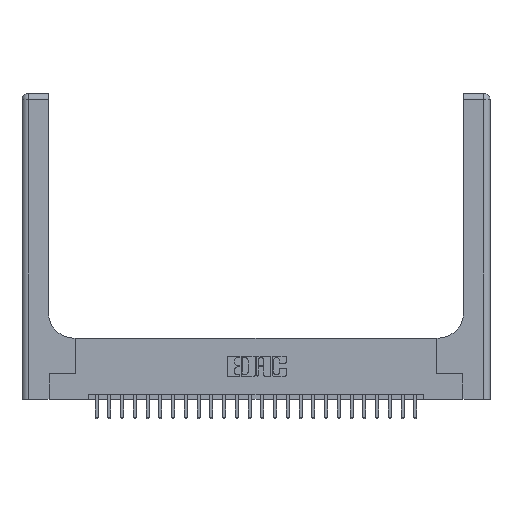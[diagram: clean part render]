
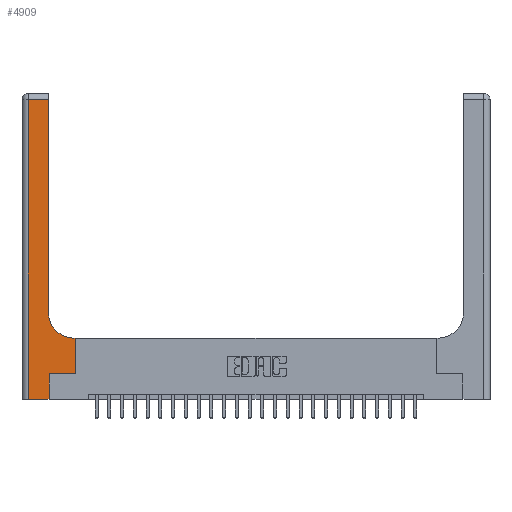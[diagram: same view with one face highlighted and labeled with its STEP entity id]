
A CAD part, top view. The second image highlights one B-rep face of the part: STEP entity #4909.
In plain terms, the highlighted planar face has unit normal (0, 0, 1).
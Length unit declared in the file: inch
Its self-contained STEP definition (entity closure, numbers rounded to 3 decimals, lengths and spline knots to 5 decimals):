
#277 = VERTEX_POINT ( 'NONE', #5348 ) ;
#520 = ORIENTED_EDGE ( 'NONE', *, *, #7861, .T. ) ;
#521 = EDGE_LOOP ( 'NONE', ( #4252, #520, #1349, #4184, #19137, #22256, #4974, #17528, #8665 ) ) ;
#565 = CIRCLE ( 'NONE', #12710, 0.25 ) ;
#1179 = EDGE_CURVE ( 'NONE', #9681, #13817, #15009, .T. ) ;
#1234 = LINE ( 'NONE', #13114, #2356 ) ;
#1349 = ORIENTED_EDGE ( 'NONE', *, *, #9516, .T. ) ;
#1449 = LINE ( 'NONE', #10674, #3967 ) ;
#2350 = EDGE_CURVE ( 'NONE', #13817, #20761, #4667, .T. ) ;
#2356 = VECTOR ( 'NONE', #8945, 39.37008 ) ;
#2433 = CARTESIAN_POINT ( 'NONE',  ( 0.265, 0., 0.37 ) ) ;
#2461 = CARTESIAN_POINT ( 'NONE',  ( 0.26, 2.94, 0.37 ) ) ;
#2468 = LINE ( 'NONE', #4597, #19761 ) ;
#2512 = EDGE_CURVE ( 'NONE', #20761, #14461, #565, .T. ) ;
#3032 = AXIS2_PLACEMENT_3D ( 'NONE', #6462, #14175, #21821 ) ;
#3412 = DIRECTION ( 'NONE',  ( 1., 0., 0. ) ) ;
#3967 = VECTOR ( 'NONE', #9165, 39.37008 ) ;
#4184 = ORIENTED_EDGE ( 'NONE', *, *, #15931, .T. ) ;
#4252 = ORIENTED_EDGE ( 'NONE', *, *, #15106, .T. ) ;
#4255 = VECTOR ( 'NONE', #4889, 39.37008 ) ;
#4597 = CARTESIAN_POINT ( 'NONE',  ( 0.06, 3., 0.37 ) ) ;
#4667 = LINE ( 'NONE', #8610, #19079 ) ;
#4889 = DIRECTION ( 'NONE',  ( 0., 1., 0. ) ) ;
#4909 = ADVANCED_FACE ( 'NONE', ( #14680 ), #23694, .F. ) ;
#4974 = ORIENTED_EDGE ( 'NONE', *, *, #1179, .T. ) ;
#5114 = CARTESIAN_POINT ( 'NONE',  ( 0.528, 0.25, 0.37 ) ) ;
#5348 = CARTESIAN_POINT ( 'NONE',  ( 0.06, 2.94, 0.37 ) ) ;
#5418 = CARTESIAN_POINT ( 'NONE',  ( 0.265, 0.25, 0.37 ) ) ;
#6462 = CARTESIAN_POINT ( 'NONE',  ( 0., 3., 0.37 ) ) ;
#6957 = DIRECTION ( 'NONE',  ( -1., 0., 0. ) ) ;
#7425 = DIRECTION ( 'NONE',  ( 0., 1., 0. ) ) ;
#7861 = EDGE_CURVE ( 'NONE', #8189, #277, #1234, .T. ) ;
#8189 = VERTEX_POINT ( 'NONE', #2461 ) ;
#8348 = VERTEX_POINT ( 'NONE', #12142 ) ;
#8610 = CARTESIAN_POINT ( 'NONE',  ( 0.26, 0.6, 0.37 ) ) ;
#8665 = ORIENTED_EDGE ( 'NONE', *, *, #2512, .T. ) ;
#8945 = DIRECTION ( 'NONE',  ( -1., 0., 0. ) ) ;
#9165 = DIRECTION ( 'NONE',  ( 1., 0., 0. ) ) ;
#9479 = DIRECTION ( 'NONE',  ( 0., 0., -1. ) ) ;
#9516 = EDGE_CURVE ( 'NONE', #277, #8348, #2468, .T. ) ;
#9681 = VERTEX_POINT ( 'NONE', #5114 ) ;
#10156 = LINE ( 'NONE', #15953, #14653 ) ;
#10674 = CARTESIAN_POINT ( 'NONE',  ( 0., 0., 0.37 ) ) ;
#10682 = CARTESIAN_POINT ( 'NONE',  ( 0.265, 0.25, 0.37 ) ) ;
#11364 = CARTESIAN_POINT ( 'NONE',  ( 0.51, 0.85, 0.37 ) ) ;
#12053 = DIRECTION ( 'NONE',  ( 0., 1., 0. ) ) ;
#12142 = CARTESIAN_POINT ( 'NONE',  ( 0.06, 0., 0.37 ) ) ;
#12207 = DIRECTION ( 'NONE',  ( 0., -1., 0. ) ) ;
#12710 = AXIS2_PLACEMENT_3D ( 'NONE', #11364, #9479, #3412 ) ;
#13114 = CARTESIAN_POINT ( 'NONE',  ( 0., 2.94, 0.37 ) ) ;
#13817 = VERTEX_POINT ( 'NONE', #21434 ) ;
#13982 = VECTOR ( 'NONE', #17362, 39.37008 ) ;
#14175 = DIRECTION ( 'NONE',  ( 0., 0., -1. ) ) ;
#14461 = VERTEX_POINT ( 'NONE', #16262 ) ;
#14653 = VECTOR ( 'NONE', #12053, 39.37008 ) ;
#14680 = FACE_OUTER_BOUND ( 'NONE', #521, .T. ) ;
#15009 = LINE ( 'NONE', #22634, #17061 ) ;
#15106 = EDGE_CURVE ( 'NONE', #14461, #8189, #10156, .T. ) ;
#15512 = CARTESIAN_POINT ( 'NONE',  ( 0.51, 0.6, 0.37 ) ) ;
#15931 = EDGE_CURVE ( 'NONE', #8348, #24026, #1449, .T. ) ;
#15953 = CARTESIAN_POINT ( 'NONE',  ( 0.26, 3., 0.37 ) ) ;
#16262 = CARTESIAN_POINT ( 'NONE',  ( 0.26, 0.85, 0.37 ) ) ;
#16788 = EDGE_CURVE ( 'NONE', #24026, #17146, #22136, .T. ) ;
#17061 = VECTOR ( 'NONE', #7425, 39.37008 ) ;
#17146 = VERTEX_POINT ( 'NONE', #10682 ) ;
#17362 = DIRECTION ( 'NONE',  ( 1., 0., 0. ) ) ;
#17528 = ORIENTED_EDGE ( 'NONE', *, *, #2350, .T. ) ;
#18492 = CARTESIAN_POINT ( 'NONE',  ( 0.265, 0., 0.37 ) ) ;
#19079 = VECTOR ( 'NONE', #6957, 39.37008 ) ;
#19137 = ORIENTED_EDGE ( 'NONE', *, *, #16788, .T. ) ;
#19215 = EDGE_CURVE ( 'NONE', #17146, #9681, #19485, .T. ) ;
#19485 = LINE ( 'NONE', #5418, #13982 ) ;
#19761 = VECTOR ( 'NONE', #12207, 39.37008 ) ;
#20761 = VERTEX_POINT ( 'NONE', #15512 ) ;
#21434 = CARTESIAN_POINT ( 'NONE',  ( 0.528, 0.6, 0.37 ) ) ;
#21821 = DIRECTION ( 'NONE',  ( -1., 0., 0. ) ) ;
#22136 = LINE ( 'NONE', #18492, #4255 ) ;
#22256 = ORIENTED_EDGE ( 'NONE', *, *, #19215, .T. ) ;
#22634 = CARTESIAN_POINT ( 'NONE',  ( 0.528, 0.25, 0.37 ) ) ;
#23694 = PLANE ( 'NONE',  #3032 ) ;
#24026 = VERTEX_POINT ( 'NONE', #2433 ) ;
